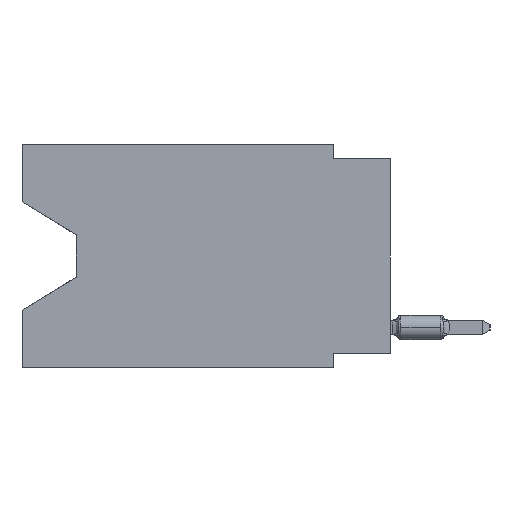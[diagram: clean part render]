
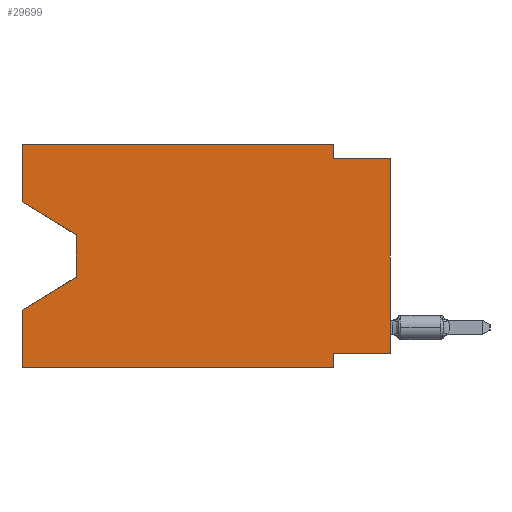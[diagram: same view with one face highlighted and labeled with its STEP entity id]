
A CAD part, left-side view. The second image highlights one B-rep face of the part: STEP entity #29699.
In plain terms, the highlighted planar face has unit normal (-1, 0, 0).
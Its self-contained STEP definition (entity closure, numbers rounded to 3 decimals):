
#615 = LINE ( 'NONE', #57451, #23096 ) ;
#933 = DIRECTION ( 'NONE',  ( 0., -0.855, -0.519 ) ) ;
#1192 = DIRECTION ( 'NONE',  ( 1., 0., 0. ) ) ;
#1267 = CARTESIAN_POINT ( 'NONE',  ( 0., 16.383, 0. ) ) ;
#1614 = EDGE_CURVE ( 'NONE', #19959, #3964, #615, .T. ) ;
#1805 = VERTEX_POINT ( 'NONE', #7498 ) ;
#3639 = DIRECTION ( 'NONE',  ( 0., -1., 0. ) ) ;
#3964 = VERTEX_POINT ( 'NONE', #17905 ) ;
#4167 = VECTOR ( 'NONE', #8638, 1000. ) ;
#4663 = ORIENTED_EDGE ( 'NONE', *, *, #14807, .F. ) ;
#4956 = VECTOR ( 'NONE', #58729, 1000. ) ;
#5299 = CARTESIAN_POINT ( 'NONE',  ( 0., 2.54, 0. ) ) ;
#5896 = FACE_OUTER_BOUND ( 'NONE', #37160, .T. ) ;
#6280 = VERTEX_POINT ( 'NONE', #27109 ) ;
#7461 = CARTESIAN_POINT ( 'NONE',  ( 0., 16.383, 0. ) ) ;
#7498 = CARTESIAN_POINT ( 'NONE',  ( 0., 0., -9.271 ) ) ;
#7947 = CARTESIAN_POINT ( 'NONE',  ( 0., 0., -9.271 ) ) ;
#8064 = ORIENTED_EDGE ( 'NONE', *, *, #61979, .F. ) ;
#8638 = DIRECTION ( 'NONE',  ( 0., 0., 1. ) ) ;
#8710 = EDGE_CURVE ( 'NONE', #53225, #6280, #31345, .T. ) ;
#8749 = CARTESIAN_POINT ( 'NONE',  ( 0., 2.54, -9.906 ) ) ;
#9697 = CARTESIAN_POINT ( 'NONE',  ( 0., 13.97, -4.013 ) ) ;
#10496 = ORIENTED_EDGE ( 'NONE', *, *, #55469, .F. ) ;
#11036 = VECTOR ( 'NONE', #23549, 1000. ) ;
#11268 = EDGE_CURVE ( 'NONE', #14214, #47211, #60689, .T. ) ;
#12130 = LINE ( 'NONE', #55159, #32188 ) ;
#12180 = VECTOR ( 'NONE', #24473, 1000. ) ;
#12345 = VECTOR ( 'NONE', #18298, 1000. ) ;
#12608 = ORIENTED_EDGE ( 'NONE', *, *, #11268, .F. ) ;
#13069 = CARTESIAN_POINT ( 'NONE',  ( 0., 16.383, -9.906 ) ) ;
#13925 = CARTESIAN_POINT ( 'NONE',  ( 0., 16.383, -2.546 ) ) ;
#14214 = VERTEX_POINT ( 'NONE', #19365 ) ;
#14807 = EDGE_CURVE ( 'NONE', #36406, #14214, #42479, .T. ) ;
#17169 = DIRECTION ( 'NONE',  ( 0., 0., -1. ) ) ;
#17787 = CARTESIAN_POINT ( 'NONE',  ( 0., 0., -0.635 ) ) ;
#17905 = CARTESIAN_POINT ( 'NONE',  ( 0., 13.97, -4.013 ) ) ;
#18298 = DIRECTION ( 'NONE',  ( 0., -1., 0. ) ) ;
#19290 = CARTESIAN_POINT ( 'NONE',  ( 0., 0., 0. ) ) ;
#19365 = CARTESIAN_POINT ( 'NONE',  ( 0., 2.54, 0. ) ) ;
#19959 = VERTEX_POINT ( 'NONE', #13925 ) ;
#20582 = CARTESIAN_POINT ( 'NONE',  ( 0., 16.383, -9.906 ) ) ;
#21208 = ORIENTED_EDGE ( 'NONE', *, *, #22098, .T. ) ;
#21611 = DIRECTION ( 'NONE',  ( 0., -1., 0. ) ) ;
#22083 = DIRECTION ( 'NONE',  ( 0., 1., 0. ) ) ;
#22098 = EDGE_CURVE ( 'NONE', #23585, #6280, #36836, .T. ) ;
#22884 = EDGE_CURVE ( 'NONE', #1805, #29914, #46938, .T. ) ;
#23096 = VECTOR ( 'NONE', #933, 1000. ) ;
#23549 = DIRECTION ( 'NONE',  ( 0., 0., -1. ) ) ;
#23585 = VERTEX_POINT ( 'NONE', #54814 ) ;
#24473 = DIRECTION ( 'NONE',  ( 0., 0., -1. ) ) ;
#25044 = VECTOR ( 'NONE', #36363, 1000. ) ;
#25085 = CARTESIAN_POINT ( 'NONE',  ( 0., 16.383, 0. ) ) ;
#25391 = DIRECTION ( 'NONE',  ( 0., 0., -1. ) ) ;
#26110 = ORIENTED_EDGE ( 'NONE', *, *, #42518, .F. ) ;
#27109 = CARTESIAN_POINT ( 'NONE',  ( 0., 16.383, -7.36 ) ) ;
#29699 = ADVANCED_FACE ( 'NONE', ( #5896 ), #39810, .F. ) ;
#29914 = VERTEX_POINT ( 'NONE', #17787 ) ;
#31345 = LINE ( 'NONE', #7461, #25044 ) ;
#31359 = LINE ( 'NONE', #45474, #44787 ) ;
#32188 = VECTOR ( 'NONE', #17169, 1000. ) ;
#32233 = ORIENTED_EDGE ( 'NONE', *, *, #43580, .T. ) ;
#34473 = ORIENTED_EDGE ( 'NONE', *, *, #1614, .T. ) ;
#35155 = ORIENTED_EDGE ( 'NONE', *, *, #53129, .T. ) ;
#36363 = DIRECTION ( 'NONE',  ( 0., 0., 1. ) ) ;
#36406 = VERTEX_POINT ( 'NONE', #61867 ) ;
#36836 = LINE ( 'NONE', #52182, #58243 ) ;
#37160 = EDGE_LOOP ( 'NONE', ( #34473, #32233, #21208, #61586, #35155, #47603, #26110, #57853, #8064, #12608, #4663, #10496 ) ) ;
#38288 = LINE ( 'NONE', #9697, #11036 ) ;
#39810 = PLANE ( 'NONE',  #49736 ) ;
#39880 = LINE ( 'NONE', #1267, #4956 ) ;
#41100 = VERTEX_POINT ( 'NONE', #58212 ) ;
#41955 = LINE ( 'NONE', #13069, #56998 ) ;
#42479 = LINE ( 'NONE', #55982, #12345 ) ;
#42518 = EDGE_CURVE ( 'NONE', #1805, #41100, #60708, .T. ) ;
#42975 = CARTESIAN_POINT ( 'NONE',  ( 0., 2.54, -0.635 ) ) ;
#43580 = EDGE_CURVE ( 'NONE', #3964, #23585, #38288, .T. ) ;
#44787 = VECTOR ( 'NONE', #21611, 1000. ) ;
#45474 = CARTESIAN_POINT ( 'NONE',  ( 0., 0., -0.635 ) ) ;
#46938 = LINE ( 'NONE', #19290, #4167 ) ;
#47211 = VERTEX_POINT ( 'NONE', #42975 ) ;
#47603 = ORIENTED_EDGE ( 'NONE', *, *, #56274, .F. ) ;
#49736 = AXIS2_PLACEMENT_3D ( 'NONE', #25085, #1192, #25391 ) ;
#51569 = DIRECTION ( 'NONE',  ( 0., 0.855, -0.519 ) ) ;
#52182 = CARTESIAN_POINT ( 'NONE',  ( 0., 13.97, -5.893 ) ) ;
#53129 = EDGE_CURVE ( 'NONE', #53225, #53914, #41955, .T. ) ;
#53225 = VERTEX_POINT ( 'NONE', #20582 ) ;
#53914 = VERTEX_POINT ( 'NONE', #8749 ) ;
#54814 = CARTESIAN_POINT ( 'NONE',  ( 0., 13.97, -5.893 ) ) ;
#55159 = CARTESIAN_POINT ( 'NONE',  ( 0., 2.54, -9.906 ) ) ;
#55469 = EDGE_CURVE ( 'NONE', #19959, #36406, #39880, .T. ) ;
#55982 = CARTESIAN_POINT ( 'NONE',  ( 0., 16.383, 0. ) ) ;
#56274 = EDGE_CURVE ( 'NONE', #41100, #53914, #12130, .T. ) ;
#56998 = VECTOR ( 'NONE', #3639, 1000. ) ;
#57057 = VECTOR ( 'NONE', #22083, 1000. ) ;
#57451 = CARTESIAN_POINT ( 'NONE',  ( 0., 16.383, -2.546 ) ) ;
#57853 = ORIENTED_EDGE ( 'NONE', *, *, #22884, .T. ) ;
#58212 = CARTESIAN_POINT ( 'NONE',  ( 0., 2.54, -9.271 ) ) ;
#58243 = VECTOR ( 'NONE', #51569, 1000. ) ;
#58729 = DIRECTION ( 'NONE',  ( 0., 0., 1. ) ) ;
#60689 = LINE ( 'NONE', #5299, #12180 ) ;
#60708 = LINE ( 'NONE', #7947, #57057 ) ;
#61586 = ORIENTED_EDGE ( 'NONE', *, *, #8710, .F. ) ;
#61867 = CARTESIAN_POINT ( 'NONE',  ( 0., 16.383, 0. ) ) ;
#61979 = EDGE_CURVE ( 'NONE', #47211, #29914, #31359, .T. ) ;
